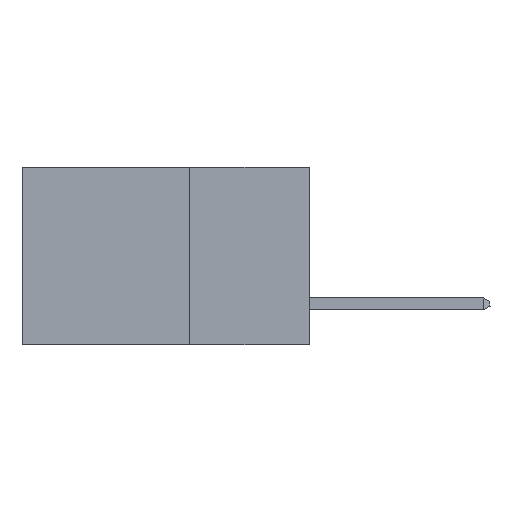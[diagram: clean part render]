
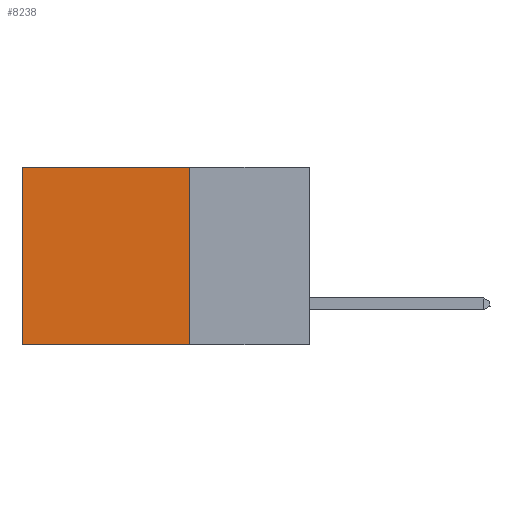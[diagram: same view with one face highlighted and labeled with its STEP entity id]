
A CAD part, left-side view. The second image highlights one B-rep face of the part: STEP entity #8238.
In plain terms, the highlighted planar face has unit normal (-1, 0, 0).
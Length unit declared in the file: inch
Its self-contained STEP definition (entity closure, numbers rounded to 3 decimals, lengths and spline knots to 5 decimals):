
#640 = VECTOR ( 'NONE', #33956, 39.37008 ) ;
#3418 = EDGE_CURVE ( 'NONE', #35182, #17065, #15927, .T. ) ;
#5187 = VECTOR ( 'NONE', #25066, 39.37008 ) ;
#7252 = CARTESIAN_POINT ( 'NONE',  ( 0.2875, 0.25, 0. ) ) ;
#7398 = AXIS2_PLACEMENT_3D ( 'NONE', #30258, #33460, #11488 ) ;
#7522 = VERTEX_POINT ( 'NONE', #38271 ) ;
#8238 = ADVANCED_FACE ( 'NONE', ( #17963 ), #17797, .F. ) ;
#8488 = DIRECTION ( 'NONE',  ( 0., 0., -1. ) ) ;
#8645 = CARTESIAN_POINT ( 'NONE',  ( 0.2875, 0.6, 0. ) ) ;
#10992 = ORIENTED_EDGE ( 'NONE', *, *, #31367, .F. ) ;
#11488 = DIRECTION ( 'NONE',  ( 0., 0., -1. ) ) ;
#11954 = CARTESIAN_POINT ( 'NONE',  ( 0.2875, 0.25, 0. ) ) ;
#13325 = LINE ( 'NONE', #35555, #37497 ) ;
#13812 = LINE ( 'NONE', #7252, #40468 ) ;
#15920 = VERTEX_POINT ( 'NONE', #27611 ) ;
#15927 = LINE ( 'NONE', #11954, #640 ) ;
#17065 = VERTEX_POINT ( 'NONE', #8645 ) ;
#17089 = DIRECTION ( 'NONE',  ( 0., 0., -1. ) ) ;
#17797 = PLANE ( 'NONE',  #7398 ) ;
#17963 = FACE_OUTER_BOUND ( 'NONE', #23840, .T. ) ;
#18727 = CARTESIAN_POINT ( 'NONE',  ( 0.2875, 0.25, 0. ) ) ;
#19312 = ORIENTED_EDGE ( 'NONE', *, *, #23568, .T. ) ;
#23568 = EDGE_CURVE ( 'NONE', #17065, #7522, #13325, .T. ) ;
#23840 = EDGE_LOOP ( 'NONE', ( #19312, #10992, #38890, #23921 ) ) ;
#23921 = ORIENTED_EDGE ( 'NONE', *, *, #3418, .T. ) ;
#25066 = DIRECTION ( 'NONE',  ( 0., 1., 0. ) ) ;
#27611 = CARTESIAN_POINT ( 'NONE',  ( 0.2875, 0.25, -0.37 ) ) ;
#28335 = EDGE_CURVE ( 'NONE', #35182, #15920, #13812, .T. ) ;
#30258 = CARTESIAN_POINT ( 'NONE',  ( 0.2875, 0.25, 0. ) ) ;
#31367 = EDGE_CURVE ( 'NONE', #15920, #7522, #32263, .T. ) ;
#32263 = LINE ( 'NONE', #34330, #5187 ) ;
#33460 = DIRECTION ( 'NONE',  ( 1., 0., 0. ) ) ;
#33956 = DIRECTION ( 'NONE',  ( 0., 1., 0. ) ) ;
#34330 = CARTESIAN_POINT ( 'NONE',  ( 0.2875, 0.25, -0.37 ) ) ;
#35182 = VERTEX_POINT ( 'NONE', #18727 ) ;
#35555 = CARTESIAN_POINT ( 'NONE',  ( 0.2875, 0.6, 0. ) ) ;
#37497 = VECTOR ( 'NONE', #17089, 39.37008 ) ;
#38271 = CARTESIAN_POINT ( 'NONE',  ( 0.2875, 0.6, -0.37 ) ) ;
#38890 = ORIENTED_EDGE ( 'NONE', *, *, #28335, .F. ) ;
#40468 = VECTOR ( 'NONE', #8488, 39.37008 ) ;
